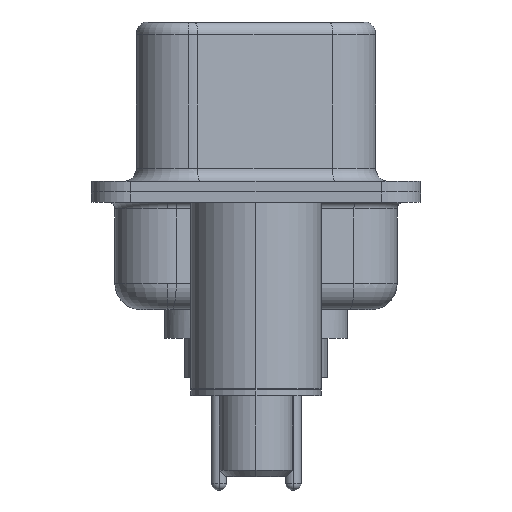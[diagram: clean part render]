
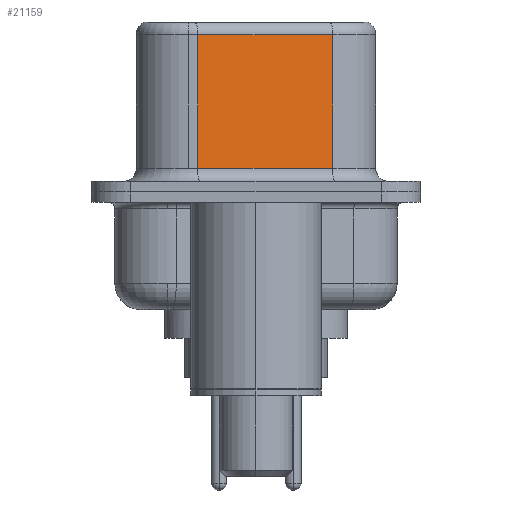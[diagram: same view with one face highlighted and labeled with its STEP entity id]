
A CAD part, left-side view. The second image highlights one B-rep face of the part: STEP entity #21159.
In plain terms, the highlighted planar face has unit normal (-0.985, -0.174, 0).
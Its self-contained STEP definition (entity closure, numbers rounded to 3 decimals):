
#346 = EDGE_LOOP ( 'NONE', ( #20773, #12437, #13115, #14287 ) ) ;
#1628 = DIRECTION ( 'NONE',  ( 0.174, -0.985, 0. ) ) ;
#4981 = CARTESIAN_POINT ( 'NONE',  ( 4.585, -2.927, 6.02 ) ) ;
#6020 = LINE ( 'NONE', #20564, #19214 ) ;
#7281 = CARTESIAN_POINT ( 'NONE',  ( 4.585, -2.927, 6.52 ) ) ;
#7528 = EDGE_CURVE ( 'NONE', #10876, #20309, #13922, .T. ) ;
#8670 = LINE ( 'NONE', #21248, #12622 ) ;
#9475 = VECTOR ( 'NONE', #19882, 1000. ) ;
#9658 = DIRECTION ( 'NONE',  ( 0., 0., -1. ) ) ;
#10519 = EDGE_CURVE ( 'NONE', #10876, #15815, #8670, .T. ) ;
#10549 = EDGE_CURVE ( 'NONE', #16619, #15815, #16449, .T. ) ;
#10822 = CARTESIAN_POINT ( 'NONE',  ( 4.585, -2.927, 6.02 ) ) ;
#10876 = VERTEX_POINT ( 'NONE', #10822 ) ;
#12096 = VECTOR ( 'NONE', #1628, 1000. ) ;
#12437 = ORIENTED_EDGE ( 'NONE', *, *, #7528, .T. ) ;
#12484 = DIRECTION ( 'NONE',  ( 0., 0., -1. ) ) ;
#12622 = VECTOR ( 'NONE', #9658, 1000. ) ;
#12974 = CARTESIAN_POINT ( 'NONE',  ( 3.675, 2.233, 0.9 ) ) ;
#13115 = ORIENTED_EDGE ( 'NONE', *, *, #16433, .T. ) ;
#13922 = LINE ( 'NONE', #4981, #9475 ) ;
#13974 = CARTESIAN_POINT ( 'NONE',  ( 3.675, 2.233, 6.02 ) ) ;
#14287 = ORIENTED_EDGE ( 'NONE', *, *, #10549, .T. ) ;
#15765 = CARTESIAN_POINT ( 'NONE',  ( 4.585, -2.927, 0.9 ) ) ;
#15815 = VERTEX_POINT ( 'NONE', #15765 ) ;
#15948 = FACE_OUTER_BOUND ( 'NONE', #346, .T. ) ;
#16433 = EDGE_CURVE ( 'NONE', #20309, #16619, #6020, .T. ) ;
#16449 = LINE ( 'NONE', #21381, #12096 ) ;
#16608 = AXIS2_PLACEMENT_3D ( 'NONE', #7281, #17076, #18806 ) ;
#16619 = VERTEX_POINT ( 'NONE', #12974 ) ;
#17076 = DIRECTION ( 'NONE',  ( 0.985, 0.174, 0. ) ) ;
#18806 = DIRECTION ( 'NONE',  ( -0.174, 0.985, 0. ) ) ;
#19214 = VECTOR ( 'NONE', #12484, 1000. ) ;
#19882 = DIRECTION ( 'NONE',  ( -0.174, 0.985, 0. ) ) ;
#20309 = VERTEX_POINT ( 'NONE', #13974 ) ;
#20340 = PLANE ( 'NONE',  #16608 ) ;
#20564 = CARTESIAN_POINT ( 'NONE',  ( 3.675, 2.233, 6.52 ) ) ;
#20773 = ORIENTED_EDGE ( 'NONE', *, *, #10519, .F. ) ;
#21159 = ADVANCED_FACE ( 'NONE', ( #15948 ), #20340, .F. ) ;
#21248 = CARTESIAN_POINT ( 'NONE',  ( 4.585, -2.927, 6.52 ) ) ;
#21381 = CARTESIAN_POINT ( 'NONE',  ( 4.585, -2.927, 0.9 ) ) ;
